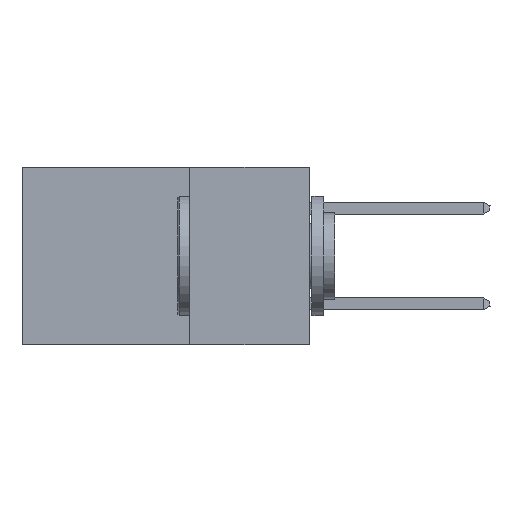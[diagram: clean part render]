
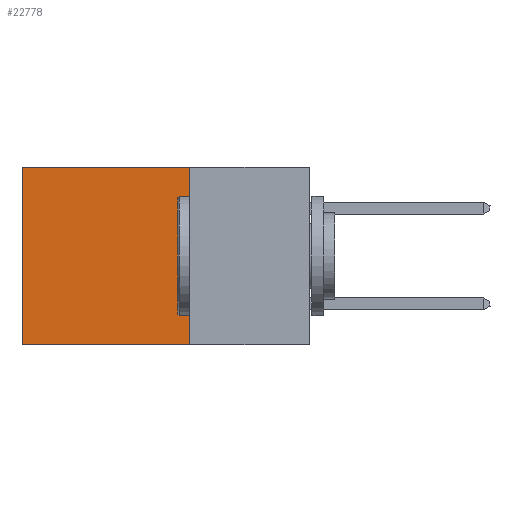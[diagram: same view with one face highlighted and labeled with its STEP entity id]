
A CAD part, left-side view. The second image highlights one B-rep face of the part: STEP entity #22778.
In plain terms, the highlighted planar face has unit normal (-1, 0, 0).
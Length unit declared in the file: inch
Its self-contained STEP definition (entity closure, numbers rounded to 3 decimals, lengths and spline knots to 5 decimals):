
#1620 = DIRECTION ( 'NONE',  ( 0., 1., 0. ) ) ;
#2829 = ORIENTED_EDGE ( 'NONE', *, *, #28606, .T. ) ;
#2879 = VECTOR ( 'NONE', #10255, 39.37008 ) ;
#3777 = CARTESIAN_POINT ( 'NONE',  ( 0.2875, 0.25, 0. ) ) ;
#4860 = CARTESIAN_POINT ( 'NONE',  ( 0.2875, 0.6, -0.37 ) ) ;
#7995 = CARTESIAN_POINT ( 'NONE',  ( 0.2875, 0.25, 0. ) ) ;
#10255 = DIRECTION ( 'NONE',  ( 0., 0., -1. ) ) ;
#10531 = PLANE ( 'NONE',  #18724 ) ;
#13134 = FACE_OUTER_BOUND ( 'NONE', #30053, .T. ) ;
#13594 = VERTEX_POINT ( 'NONE', #7995 ) ;
#14316 = VERTEX_POINT ( 'NONE', #36281 ) ;
#15274 = CARTESIAN_POINT ( 'NONE',  ( 0.2875, 0.25, -0.37 ) ) ;
#15982 = EDGE_CURVE ( 'NONE', #13594, #18181, #26464, .T. ) ;
#16221 = LINE ( 'NONE', #3777, #2879 ) ;
#17372 = DIRECTION ( 'NONE',  ( 1., 0., 0. ) ) ;
#17655 = ORIENTED_EDGE ( 'NONE', *, *, #38848, .F. ) ;
#17698 = DIRECTION ( 'NONE',  ( 0., 1., 0. ) ) ;
#17853 = VERTEX_POINT ( 'NONE', #4860 ) ;
#18181 = VERTEX_POINT ( 'NONE', #34402 ) ;
#18724 = AXIS2_PLACEMENT_3D ( 'NONE', #37775, #17372, #41201 ) ;
#20555 = LINE ( 'NONE', #25495, #36009 ) ;
#20760 = ORIENTED_EDGE ( 'NONE', *, *, #24587, .F. ) ;
#22778 = ADVANCED_FACE ( 'NONE', ( #13134 ), #10531, .F. ) ;
#24587 = EDGE_CURVE ( 'NONE', #13594, #14316, #16221, .T. ) ;
#24877 = CARTESIAN_POINT ( 'NONE',  ( 0.2875, 0.25, 0. ) ) ;
#25495 = CARTESIAN_POINT ( 'NONE',  ( 0.2875, 0.6, 0. ) ) ;
#26464 = LINE ( 'NONE', #24877, #32333 ) ;
#26701 = VECTOR ( 'NONE', #1620, 39.37008 ) ;
#28606 = EDGE_CURVE ( 'NONE', #18181, #17853, #20555, .T. ) ;
#28987 = ORIENTED_EDGE ( 'NONE', *, *, #15982, .T. ) ;
#30053 = EDGE_LOOP ( 'NONE', ( #2829, #17655, #20760, #28987 ) ) ;
#32333 = VECTOR ( 'NONE', #17698, 39.37008 ) ;
#32459 = DIRECTION ( 'NONE',  ( 0., 0., -1. ) ) ;
#34402 = CARTESIAN_POINT ( 'NONE',  ( 0.2875, 0.6, 0. ) ) ;
#35761 = LINE ( 'NONE', #15274, #26701 ) ;
#36009 = VECTOR ( 'NONE', #32459, 39.37008 ) ;
#36281 = CARTESIAN_POINT ( 'NONE',  ( 0.2875, 0.25, -0.37 ) ) ;
#37775 = CARTESIAN_POINT ( 'NONE',  ( 0.2875, 0.25, 0. ) ) ;
#38848 = EDGE_CURVE ( 'NONE', #14316, #17853, #35761, .T. ) ;
#41201 = DIRECTION ( 'NONE',  ( 0., 0., -1. ) ) ;
